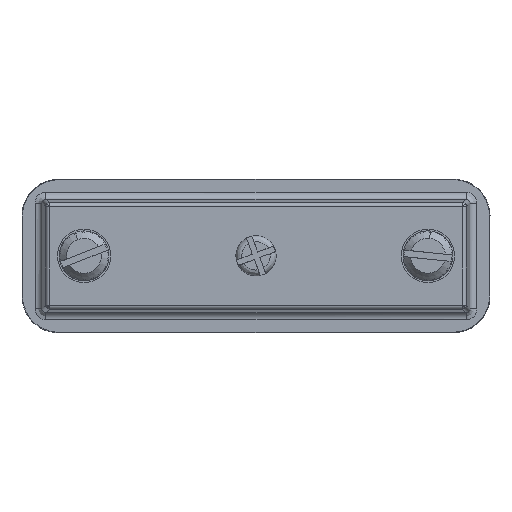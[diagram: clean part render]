
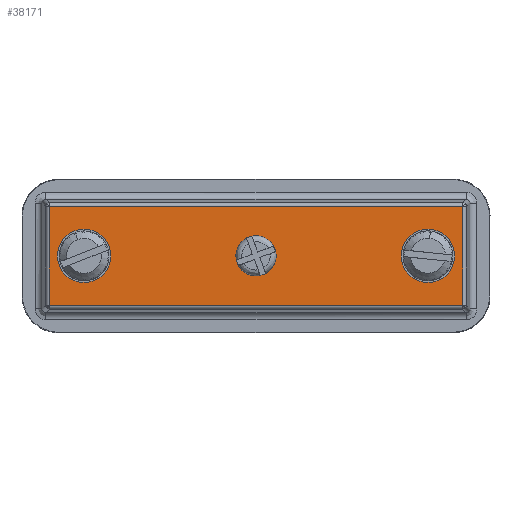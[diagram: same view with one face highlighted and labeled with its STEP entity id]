
A CAD part, top view. The second image highlights one B-rep face of the part: STEP entity #38171.
In plain terms, the highlighted planar face has unit normal (0, 0, 1).
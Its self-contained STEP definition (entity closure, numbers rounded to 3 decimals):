
#1391 = DIRECTION ( 'NONE',  ( 1., 0., 0. ) ) ;
#2272 = AXIS2_PLACEMENT_3D ( 'NONE', #28845, #5873, #16990 ) ;
#2873 = CARTESIAN_POINT ( 'NONE',  ( 0., 0., 7.5 ) ) ;
#3237 = DIRECTION ( 'NONE',  ( 0., -1., 0. ) ) ;
#3491 = CARTESIAN_POINT ( 'NONE',  ( 5.5, -3.845, 7.5 ) ) ;
#3592 = PLANE ( 'NONE',  #20086 ) ;
#3924 = VERTEX_POINT ( 'NONE', #36666 ) ;
#4082 = DIRECTION ( 'NONE',  ( 0., 0., -1. ) ) ;
#4157 = CIRCLE ( 'NONE', #25097, 3.65 ) ;
#4179 = CARTESIAN_POINT ( 'NONE',  ( 6.65, 19.675, 7.5 ) ) ;
#5001 = CARTESIAN_POINT ( 'NONE',  ( 2.377, -8.618, 7.5 ) ) ;
#5248 = CARTESIAN_POINT ( 'NONE',  ( 9.15, 19.675, 7.5 ) ) ;
#5767 = VERTEX_POINT ( 'NONE', #5001 ) ;
#5873 = DIRECTION ( 'NONE',  ( 0., 0., -1. ) ) ;
#6273 = FACE_BOUND ( 'NONE', #25604, .T. ) ;
#6448 = EDGE_LOOP ( 'NONE', ( #43040, #39302 ) ) ;
#7148 = CARTESIAN_POINT ( 'NONE',  ( 0., -8.618, 7.5 ) ) ;
#7326 = LINE ( 'NONE', #13870, #27054 ) ;
#7574 = AXIS2_PLACEMENT_3D ( 'NONE', #42026, #16864, #28242 ) ;
#7784 = EDGE_CURVE ( 'NONE', #14415, #45513, #44840, .T. ) ;
#9126 = EDGE_LOOP ( 'NONE', ( #42070, #15136 ) ) ;
#9919 = CARTESIAN_POINT ( 'NONE',  ( 2.377, 47.968, 7.5 ) ) ;
#9992 = ORIENTED_EDGE ( 'NONE', *, *, #46059, .T. ) ;
#11644 = EDGE_CURVE ( 'NONE', #45696, #35312, #15300, .T. ) ;
#11732 = CARTESIAN_POINT ( 'NONE',  ( 0., 47.968, 7.5 ) ) ;
#13453 = DIRECTION ( 'NONE',  ( 1., 0., 0. ) ) ;
#13870 = CARTESIAN_POINT ( 'NONE',  ( 2.377, 0., 7.5 ) ) ;
#14084 = AXIS2_PLACEMENT_3D ( 'NONE', #5248, #46088, #1391 ) ;
#14415 = VERTEX_POINT ( 'NONE', #40131 ) ;
#15136 = ORIENTED_EDGE ( 'NONE', *, *, #26162, .T. ) ;
#15300 = CIRCLE ( 'NONE', #7574, 3.65 ) ;
#15875 = DIRECTION ( 'NONE',  ( 0., 0., -1. ) ) ;
#16378 = AXIS2_PLACEMENT_3D ( 'NONE', #41522, #27734, #13453 ) ;
#16864 = DIRECTION ( 'NONE',  ( 0., 0., -1. ) ) ;
#16990 = DIRECTION ( 'NONE',  ( 1., 0., 0. ) ) ;
#17041 = EDGE_CURVE ( 'NONE', #35312, #45696, #31611, .T. ) ;
#18312 = ORIENTED_EDGE ( 'NONE', *, *, #42694, .T. ) ;
#18560 = VERTEX_POINT ( 'NONE', #36330 ) ;
#19111 = VECTOR ( 'NONE', #41218, 1000. ) ;
#19536 = LINE ( 'NONE', #23166, #41006 ) ;
#19571 = VERTEX_POINT ( 'NONE', #4179 ) ;
#19758 = CARTESIAN_POINT ( 'NONE',  ( 9.15, 19.675, 7.5 ) ) ;
#20086 = AXIS2_PLACEMENT_3D ( 'NONE', #2873, #47335, #46852 ) ;
#21594 = EDGE_CURVE ( 'NONE', #45513, #5767, #7326, .T. ) ;
#21675 = DIRECTION ( 'NONE',  ( 1., 0., 0. ) ) ;
#21789 = VECTOR ( 'NONE', #21675, 1000. ) ;
#22454 = DIRECTION ( 'NONE',  ( 1., 0., 0. ) ) ;
#23166 = CARTESIAN_POINT ( 'NONE',  ( 15.923, 0., 7.5 ) ) ;
#23543 = CIRCLE ( 'NONE', #14084, 2.5 ) ;
#25097 = AXIS2_PLACEMENT_3D ( 'NONE', #45136, #4082, #22454 ) ;
#25361 = ORIENTED_EDGE ( 'NONE', *, *, #11644, .T. ) ;
#25584 = CARTESIAN_POINT ( 'NONE',  ( 12.8, 43.195, 7.5 ) ) ;
#25604 = EDGE_LOOP ( 'NONE', ( #25361, #46379 ) ) ;
#26099 = EDGE_CURVE ( 'NONE', #34862, #34680, #4157, .T. ) ;
#26162 = EDGE_CURVE ( 'NONE', #19571, #3924, #23543, .T. ) ;
#27054 = VECTOR ( 'NONE', #3237, 1000. ) ;
#27734 = DIRECTION ( 'NONE',  ( 0., 0., -1. ) ) ;
#27754 = CARTESIAN_POINT ( 'NONE',  ( 5.5, 43.195, 7.5 ) ) ;
#28242 = DIRECTION ( 'NONE',  ( 1., 0., 0. ) ) ;
#28759 = AXIS2_PLACEMENT_3D ( 'NONE', #19758, #15875, #31131 ) ;
#28845 = CARTESIAN_POINT ( 'NONE',  ( 9.15, 43.195, 7.5 ) ) ;
#29480 = FACE_BOUND ( 'NONE', #9126, .T. ) ;
#30663 = DIRECTION ( 'NONE',  ( 0., 1., 0. ) ) ;
#31131 = DIRECTION ( 'NONE',  ( 1., 0., 0. ) ) ;
#31611 = CIRCLE ( 'NONE', #2272, 3.65 ) ;
#34680 = VERTEX_POINT ( 'NONE', #34708 ) ;
#34708 = CARTESIAN_POINT ( 'NONE',  ( 12.8, -3.845, 7.5 ) ) ;
#34862 = VERTEX_POINT ( 'NONE', #3491 ) ;
#35312 = VERTEX_POINT ( 'NONE', #27754 ) ;
#35581 = CIRCLE ( 'NONE', #16378, 3.65 ) ;
#36330 = CARTESIAN_POINT ( 'NONE',  ( 15.923, -8.618, 7.5 ) ) ;
#36666 = CARTESIAN_POINT ( 'NONE',  ( 11.65, 19.675, 7.5 ) ) ;
#37966 = ORIENTED_EDGE ( 'NONE', *, *, #7784, .T. ) ;
#38171 = ADVANCED_FACE ( 'NONE', ( #29480, #43247, #6273, #39625 ), #3592, .T. ) ;
#39302 = ORIENTED_EDGE ( 'NONE', *, *, #26099, .T. ) ;
#39625 = FACE_OUTER_BOUND ( 'NONE', #40734, .T. ) ;
#40131 = CARTESIAN_POINT ( 'NONE',  ( 15.923, 47.968, 7.5 ) ) ;
#40734 = EDGE_LOOP ( 'NONE', ( #18312, #37966, #47668, #9992 ) ) ;
#41006 = VECTOR ( 'NONE', #30663, 1000. ) ;
#41218 = DIRECTION ( 'NONE',  ( -1., 0., 0. ) ) ;
#41522 = CARTESIAN_POINT ( 'NONE',  ( 9.15, -3.845, 7.5 ) ) ;
#42026 = CARTESIAN_POINT ( 'NONE',  ( 9.15, 43.195, 7.5 ) ) ;
#42070 = ORIENTED_EDGE ( 'NONE', *, *, #46793, .T. ) ;
#42535 = CIRCLE ( 'NONE', #28759, 2.5 ) ;
#42694 = EDGE_CURVE ( 'NONE', #18560, #14415, #19536, .T. ) ;
#43040 = ORIENTED_EDGE ( 'NONE', *, *, #46868, .T. ) ;
#43247 = FACE_BOUND ( 'NONE', #6448, .T. ) ;
#43421 = LINE ( 'NONE', #7148, #21789 ) ;
#44840 = LINE ( 'NONE', #11732, #19111 ) ;
#45136 = CARTESIAN_POINT ( 'NONE',  ( 9.15, -3.845, 7.5 ) ) ;
#45513 = VERTEX_POINT ( 'NONE', #9919 ) ;
#45696 = VERTEX_POINT ( 'NONE', #25584 ) ;
#46059 = EDGE_CURVE ( 'NONE', #5767, #18560, #43421, .T. ) ;
#46088 = DIRECTION ( 'NONE',  ( 0., 0., -1. ) ) ;
#46379 = ORIENTED_EDGE ( 'NONE', *, *, #17041, .T. ) ;
#46793 = EDGE_CURVE ( 'NONE', #3924, #19571, #42535, .T. ) ;
#46852 = DIRECTION ( 'NONE',  ( 1., 0., 0. ) ) ;
#46868 = EDGE_CURVE ( 'NONE', #34680, #34862, #35581, .T. ) ;
#47335 = DIRECTION ( 'NONE',  ( 0., 0., 1. ) ) ;
#47668 = ORIENTED_EDGE ( 'NONE', *, *, #21594, .T. ) ;
